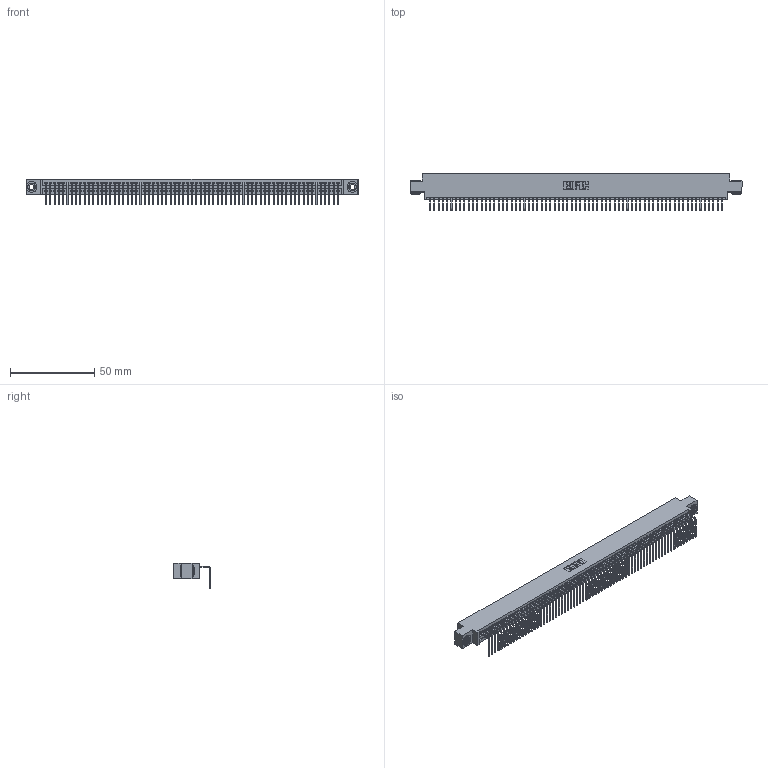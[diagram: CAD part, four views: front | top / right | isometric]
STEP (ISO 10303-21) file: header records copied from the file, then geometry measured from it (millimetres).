
FILE_DESCRIPTION (( 'STEP AP203' ), '1' );
FILE_NAME ('395-069-558-603.STEP', '2019-10-11T19:51:49', ( '' ), ( '' ), 'SwSTEP 2.0', 'SolidWorks 2016', '' );
FILE_SCHEMA (( 'CONFIG_CONTROL_DESIGN' ));
Length unit declared in the file: inch
Products named in the file (4): 345 Part_0.170 Offset - 0.156 Dia-TH; 345-250-002_345-250-002-102; 345-292-001_558 Tail - 2; 395-069-558-603
Assembly tree (72 placements, depth 2):
  395-069-558-603
    345 Part_0.170 Offset - 0.156 Dia-TH
    345-292-001_558 Tail - 2  x69
    345-250-002_345-250-002-102  x2
Bounding box: 196.47 x 21.83 x 15.37 mm (x, y, z)
Volume: 19017.9 mm3; surface area: 27331.9 mm2
Topology: 72 solids, 72 shells, 4308 faces, 12987 edges, 8562 vertices
Faces by surface type: plane 2992, cylinder 1308, cone 8
Entity records: 49162 total; most frequent: CARTESIAN_POINT 8494, ORIENTED_EDGE 8490, DIRECTION 7409, EDGE_CURVE 4245, VECTOR 3813, LINE 3813, VERTEX_POINT 2826, AXIS2_PLACEMENT_3D 1798
